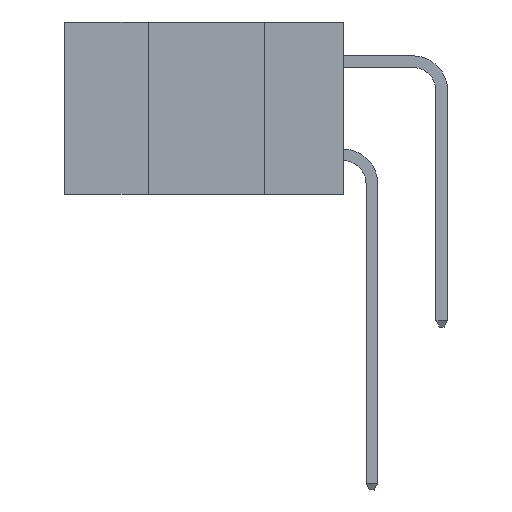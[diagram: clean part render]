
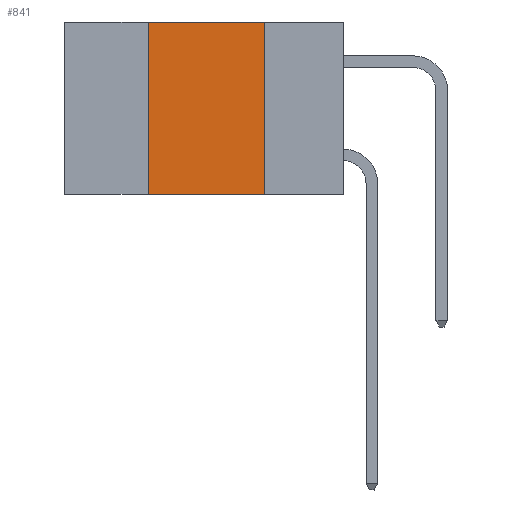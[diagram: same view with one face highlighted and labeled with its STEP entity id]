
A CAD part, left-side view. The second image highlights one B-rep face of the part: STEP entity #841.
In plain terms, the highlighted planar face has unit normal (-1, 0, 0).
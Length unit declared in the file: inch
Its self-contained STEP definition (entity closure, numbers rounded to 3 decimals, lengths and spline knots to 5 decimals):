
#84 = CARTESIAN_POINT ( 'NONE',  ( 0., 0.6, -0.37 ) ) ;
#576 = DIRECTION ( 'NONE',  ( 0., -1., 0. ) ) ;
#841 = ADVANCED_FACE ( 'NONE', ( #12691 ), #3612, .F. ) ;
#1209 = CARTESIAN_POINT ( 'NONE',  ( 0., 0.17, 0. ) ) ;
#2259 = AXIS2_PLACEMENT_3D ( 'NONE', #12217, #12117, #22640 ) ;
#2534 = EDGE_LOOP ( 'NONE', ( #4937, #14256, #6563, #7094 ) ) ;
#3612 = PLANE ( 'NONE',  #2259 ) ;
#4850 = LINE ( 'NONE', #25613, #23784 ) ;
#4937 = ORIENTED_EDGE ( 'NONE', *, *, #22872, .F. ) ;
#5855 = CARTESIAN_POINT ( 'NONE',  ( 0., 0.42, 0. ) ) ;
#6563 = ORIENTED_EDGE ( 'NONE', *, *, #17070, .F. ) ;
#6761 = VERTEX_POINT ( 'NONE', #5855 ) ;
#7094 = ORIENTED_EDGE ( 'NONE', *, *, #11192, .T. ) ;
#7496 = CARTESIAN_POINT ( 'NONE',  ( 0., 0.6, 0. ) ) ;
#8803 = VECTOR ( 'NONE', #576, 39.37008 ) ;
#11192 = EDGE_CURVE ( 'NONE', #16214, #11687, #12558, .T. ) ;
#11687 = VERTEX_POINT ( 'NONE', #20639 ) ;
#12040 = DIRECTION ( 'NONE',  ( 0., 0., -1. ) ) ;
#12117 = DIRECTION ( 'NONE',  ( 1., 0., 0. ) ) ;
#12217 = CARTESIAN_POINT ( 'NONE',  ( 0., 0.6, 0. ) ) ;
#12558 = LINE ( 'NONE', #84, #8803 ) ;
#12665 = DIRECTION ( 'NONE',  ( 0., 0., 1. ) ) ;
#12691 = FACE_OUTER_BOUND ( 'NONE', #2534, .T. ) ;
#14256 = ORIENTED_EDGE ( 'NONE', *, *, #21940, .F. ) ;
#15228 = LINE ( 'NONE', #7496, #26033 ) ;
#15902 = CARTESIAN_POINT ( 'NONE',  ( 0., 0.42, -0.37 ) ) ;
#16146 = VECTOR ( 'NONE', #12040, 39.37008 ) ;
#16214 = VERTEX_POINT ( 'NONE', #15902 ) ;
#16686 = VERTEX_POINT ( 'NONE', #1209 ) ;
#17070 = EDGE_CURVE ( 'NONE', #16214, #6761, #4850, .T. ) ;
#18830 = LINE ( 'NONE', #25015, #16146 ) ;
#20639 = CARTESIAN_POINT ( 'NONE',  ( 0., 0.17, -0.37 ) ) ;
#21940 = EDGE_CURVE ( 'NONE', #6761, #16686, #15228, .T. ) ;
#22640 = DIRECTION ( 'NONE',  ( 0., 0., -1. ) ) ;
#22652 = DIRECTION ( 'NONE',  ( 0., -1., 0. ) ) ;
#22872 = EDGE_CURVE ( 'NONE', #16686, #11687, #18830, .T. ) ;
#23784 = VECTOR ( 'NONE', #12665, 39.37008 ) ;
#25015 = CARTESIAN_POINT ( 'NONE',  ( 0., 0.17, 0. ) ) ;
#25613 = CARTESIAN_POINT ( 'NONE',  ( 0., 0.42, 0. ) ) ;
#26033 = VECTOR ( 'NONE', #22652, 39.37008 ) ;
